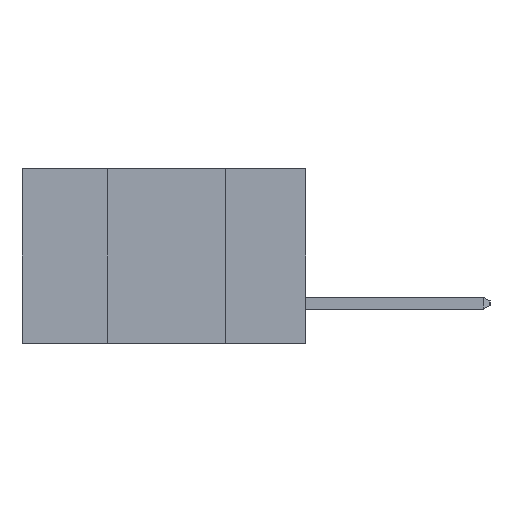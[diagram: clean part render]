
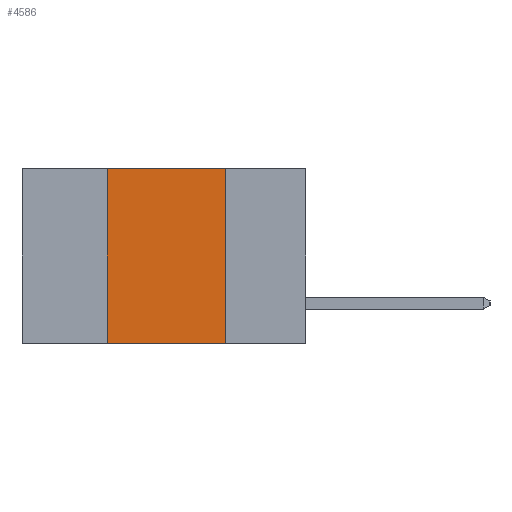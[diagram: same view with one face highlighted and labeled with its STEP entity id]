
A CAD part, left-side view. The second image highlights one B-rep face of the part: STEP entity #4586.
In plain terms, the highlighted planar face has unit normal (-1, 0, 0).
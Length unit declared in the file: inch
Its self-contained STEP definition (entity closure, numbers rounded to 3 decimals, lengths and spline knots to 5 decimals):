
#15 = LINE ( 'NONE', #5103, #6729 ) ;
#102 = CARTESIAN_POINT ( 'NONE',  ( 0., 0.17, -0.37 ) ) ;
#338 = CARTESIAN_POINT ( 'NONE',  ( 0., 0.6, -0.37 ) ) ;
#413 = DIRECTION ( 'NONE',  ( 0., -1., 0. ) ) ;
#630 = EDGE_CURVE ( 'NONE', #1315, #6942, #2149, .T. ) ;
#683 = EDGE_CURVE ( 'NONE', #4898, #4021, #15, .T. ) ;
#704 = ORIENTED_EDGE ( 'NONE', *, *, #5658, .T. ) ;
#1212 = VECTOR ( 'NONE', #4291, 39.37008 ) ;
#1315 = VERTEX_POINT ( 'NONE', #1678 ) ;
#1331 = EDGE_LOOP ( 'NONE', ( #6406, #6934, #5016, #704 ) ) ;
#1678 = CARTESIAN_POINT ( 'NONE',  ( 0., 0.17, 0. ) ) ;
#1961 = VECTOR ( 'NONE', #413, 39.37008 ) ;
#2149 = LINE ( 'NONE', #6322, #5443 ) ;
#2367 = CARTESIAN_POINT ( 'NONE',  ( 0., 0.42, 0. ) ) ;
#3069 = AXIS2_PLACEMENT_3D ( 'NONE', #6549, #6547, #6527 ) ;
#3393 = FACE_OUTER_BOUND ( 'NONE', #1331, .T. ) ;
#3733 = EDGE_CURVE ( 'NONE', #4021, #1315, #4548, .T. ) ;
#4021 = VERTEX_POINT ( 'NONE', #2367 ) ;
#4262 = CARTESIAN_POINT ( 'NONE',  ( 0., 0.6, 0. ) ) ;
#4291 = DIRECTION ( 'NONE',  ( 0., -1., 0. ) ) ;
#4548 = LINE ( 'NONE', #4262, #1212 ) ;
#4586 = ADVANCED_FACE ( 'NONE', ( #3393 ), #6573, .F. ) ;
#4898 = VERTEX_POINT ( 'NONE', #5125 ) ;
#5016 = ORIENTED_EDGE ( 'NONE', *, *, #683, .F. ) ;
#5103 = CARTESIAN_POINT ( 'NONE',  ( 0., 0.42, -0.37 ) ) ;
#5125 = CARTESIAN_POINT ( 'NONE',  ( 0., 0.42, -0.37 ) ) ;
#5339 = DIRECTION ( 'NONE',  ( 0., 0., -1. ) ) ;
#5443 = VECTOR ( 'NONE', #5339, 39.37008 ) ;
#5658 = EDGE_CURVE ( 'NONE', #4898, #6942, #5675, .T. ) ;
#5675 = LINE ( 'NONE', #338, #1961 ) ;
#6322 = CARTESIAN_POINT ( 'NONE',  ( 0., 0.17, -0.37 ) ) ;
#6406 = ORIENTED_EDGE ( 'NONE', *, *, #630, .F. ) ;
#6527 = DIRECTION ( 'NONE',  ( 0., 0., -1. ) ) ;
#6547 = DIRECTION ( 'NONE',  ( 1., 0., 0. ) ) ;
#6549 = CARTESIAN_POINT ( 'NONE',  ( 0., 0.6, 0. ) ) ;
#6573 = PLANE ( 'NONE',  #3069 ) ;
#6729 = VECTOR ( 'NONE', #7723, 39.37008 ) ;
#6934 = ORIENTED_EDGE ( 'NONE', *, *, #3733, .F. ) ;
#6942 = VERTEX_POINT ( 'NONE', #102 ) ;
#7723 = DIRECTION ( 'NONE',  ( 0., 0., 1. ) ) ;
